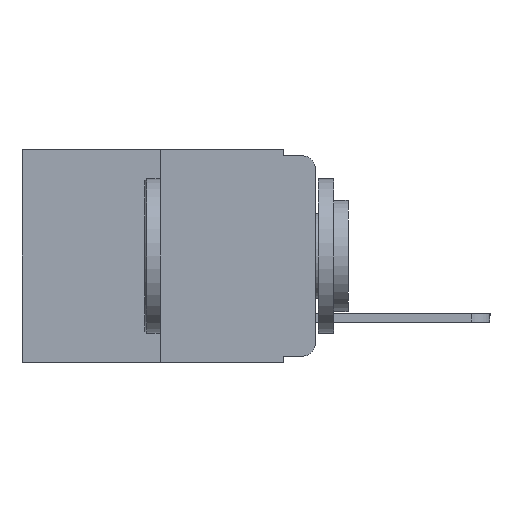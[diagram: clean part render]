
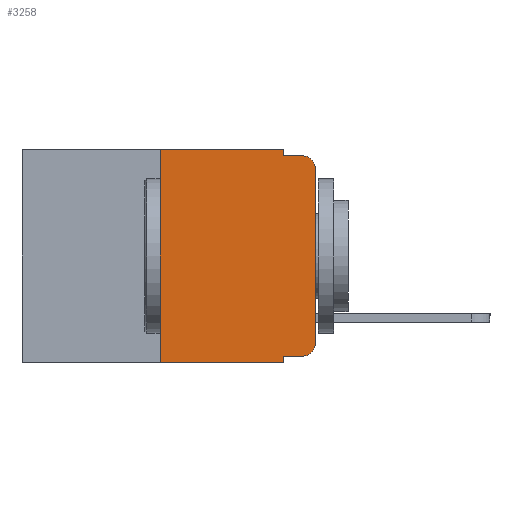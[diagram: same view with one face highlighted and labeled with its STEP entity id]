
A CAD part, left-side view. The second image highlights one B-rep face of the part: STEP entity #3258.
In plain terms, the highlighted planar face has unit normal (-1, 0, 0).
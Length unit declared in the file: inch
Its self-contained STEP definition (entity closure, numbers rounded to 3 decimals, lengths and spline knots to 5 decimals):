
#111 = VECTOR ( 'NONE', #10847, 39.37008 ) ;
#1066 = CARTESIAN_POINT ( 'NONE',  ( 0., 0.051, -0.343 ) ) ;
#1266 = AXIS2_PLACEMENT_3D ( 'NONE', #7223, #21122, #9254 ) ;
#1570 = CARTESIAN_POINT ( 'NONE',  ( 0., 0., -0.03 ) ) ;
#1697 = ORIENTED_EDGE ( 'NONE', *, *, #19129, .T. ) ;
#1716 = DIRECTION ( 'NONE',  ( 0., 0., 1. ) ) ;
#3081 = CARTESIAN_POINT ( 'NONE',  ( 0., 0.051, 0. ) ) ;
#3258 = ADVANCED_FACE ( 'NONE', ( #6547 ), #25032, .F. ) ;
#3435 = LINE ( 'NONE', #7376, #23941 ) ;
#3585 = VECTOR ( 'NONE', #14496, 39.37008 ) ;
#3629 = VECTOR ( 'NONE', #20636, 39.37008 ) ;
#4658 = VERTEX_POINT ( 'NONE', #23649 ) ;
#5950 = VECTOR ( 'NONE', #10369, 39.37008 ) ;
#6118 = ORIENTED_EDGE ( 'NONE', *, *, #22572, .T. ) ;
#6547 = FACE_OUTER_BOUND ( 'NONE', #13446, .T. ) ;
#6591 = CARTESIAN_POINT ( 'NONE',  ( 0., 0.02, -0.01 ) ) ;
#6828 = DIRECTION ( 'NONE',  ( -1., 0., 0. ) ) ;
#6910 = CARTESIAN_POINT ( 'NONE',  ( 0., 0.051, -0.333 ) ) ;
#7209 = AXIS2_PLACEMENT_3D ( 'NONE', #18781, #6828, #20740 ) ;
#7223 = CARTESIAN_POINT ( 'NONE',  ( 0., 0.02, -0.03 ) ) ;
#7250 = EDGE_CURVE ( 'NONE', #8052, #21876, #25751, .T. ) ;
#7376 = CARTESIAN_POINT ( 'NONE',  ( 0., 0.051, -0.333 ) ) ;
#7412 = LINE ( 'NONE', #8847, #111 ) ;
#7690 = ORIENTED_EDGE ( 'NONE', *, *, #24357, .F. ) ;
#7955 = LINE ( 'NONE', #3081, #17935 ) ;
#8052 = VERTEX_POINT ( 'NONE', #14837 ) ;
#8847 = CARTESIAN_POINT ( 'NONE',  ( 0., 0.051, -0.01 ) ) ;
#8939 = LINE ( 'NONE', #10450, #3585 ) ;
#8956 = ORIENTED_EDGE ( 'NONE', *, *, #12789, .F. ) ;
#9242 = DIRECTION ( 'NONE',  ( 0., -1., 0. ) ) ;
#9254 = DIRECTION ( 'NONE',  ( 0., 0., -1. ) ) ;
#9291 = EDGE_CURVE ( 'NONE', #8052, #18500, #14922, .T. ) ;
#9296 = CIRCLE ( 'NONE', #1266, 0.02 ) ;
#10038 = LINE ( 'NONE', #23091, #10674 ) ;
#10175 = ORIENTED_EDGE ( 'NONE', *, *, #10611, .F. ) ;
#10369 = DIRECTION ( 'NONE',  ( 0., -1., 0. ) ) ;
#10387 = VERTEX_POINT ( 'NONE', #17788 ) ;
#10450 = CARTESIAN_POINT ( 'NONE',  ( 0., 0.051, 0. ) ) ;
#10611 = EDGE_CURVE ( 'NONE', #18628, #21876, #8939, .T. ) ;
#10674 = VECTOR ( 'NONE', #9242, 39.37008 ) ;
#10847 = DIRECTION ( 'NONE',  ( 0., -1., 0. ) ) ;
#11144 = LINE ( 'NONE', #13752, #16442 ) ;
#11456 = ORIENTED_EDGE ( 'NONE', *, *, #21250, .T. ) ;
#12789 = EDGE_CURVE ( 'NONE', #18500, #4658, #10038, .T. ) ;
#13200 = CIRCLE ( 'NONE', #7209, 0.02 ) ;
#13446 = EDGE_LOOP ( 'NONE', ( #22276, #1697, #7690, #24114, #8956, #20131, #25324, #10175, #6118, #11456 ) ) ;
#13752 = CARTESIAN_POINT ( 'NONE',  ( 0., 0., 0. ) ) ;
#14496 = DIRECTION ( 'NONE',  ( 0., 0., -1. ) ) ;
#14837 = CARTESIAN_POINT ( 'NONE',  ( 0., 0.25, -0.343 ) ) ;
#14922 = LINE ( 'NONE', #18664, #3629 ) ;
#16130 = VERTEX_POINT ( 'NONE', #6591 ) ;
#16180 = CARTESIAN_POINT ( 'NONE',  ( 0., 0., -0.313 ) ) ;
#16442 = VECTOR ( 'NONE', #1716, 39.37008 ) ;
#16464 = EDGE_CURVE ( 'NONE', #21047, #25197, #11144, .T. ) ;
#16866 = CARTESIAN_POINT ( 'NONE',  ( 0., 0.051, -0.01 ) ) ;
#17788 = CARTESIAN_POINT ( 'NONE',  ( 0., 0.02, -0.333 ) ) ;
#17935 = VECTOR ( 'NONE', #24933, 39.37008 ) ;
#18500 = VERTEX_POINT ( 'NONE', #18513 ) ;
#18513 = CARTESIAN_POINT ( 'NONE',  ( 0., 0.25, 0. ) ) ;
#18628 = VERTEX_POINT ( 'NONE', #6910 ) ;
#18664 = CARTESIAN_POINT ( 'NONE',  ( 0., 0.25, 0. ) ) ;
#18781 = CARTESIAN_POINT ( 'NONE',  ( 0., 0.02, -0.313 ) ) ;
#19129 = EDGE_CURVE ( 'NONE', #25197, #16130, #9296, .T. ) ;
#20131 = ORIENTED_EDGE ( 'NONE', *, *, #9291, .F. ) ;
#20636 = DIRECTION ( 'NONE',  ( 0., 0., 1. ) ) ;
#20740 = DIRECTION ( 'NONE',  ( 0., 0., -1. ) ) ;
#21047 = VERTEX_POINT ( 'NONE', #16180 ) ;
#21122 = DIRECTION ( 'NONE',  ( -1., 0., 0. ) ) ;
#21250 = EDGE_CURVE ( 'NONE', #10387, #21047, #13200, .T. ) ;
#21550 = AXIS2_PLACEMENT_3D ( 'NONE', #23144, #21879, #21911 ) ;
#21876 = VERTEX_POINT ( 'NONE', #1066 ) ;
#21879 = DIRECTION ( 'NONE',  ( 1., 0., 0. ) ) ;
#21911 = DIRECTION ( 'NONE',  ( 0., 0., -1. ) ) ;
#22276 = ORIENTED_EDGE ( 'NONE', *, *, #16464, .T. ) ;
#22572 = EDGE_CURVE ( 'NONE', #18628, #10387, #3435, .T. ) ;
#23091 = CARTESIAN_POINT ( 'NONE',  ( 0., 0.473, 0. ) ) ;
#23144 = CARTESIAN_POINT ( 'NONE',  ( 0., 0.473, 0. ) ) ;
#23249 = DIRECTION ( 'NONE',  ( 0., -1., 0. ) ) ;
#23649 = CARTESIAN_POINT ( 'NONE',  ( 0., 0.051, 0. ) ) ;
#23941 = VECTOR ( 'NONE', #23249, 39.37008 ) ;
#24114 = ORIENTED_EDGE ( 'NONE', *, *, #25647, .F. ) ;
#24202 = CARTESIAN_POINT ( 'NONE',  ( 0., 0.473, -0.343 ) ) ;
#24357 = EDGE_CURVE ( 'NONE', #24376, #16130, #7412, .T. ) ;
#24376 = VERTEX_POINT ( 'NONE', #16866 ) ;
#24933 = DIRECTION ( 'NONE',  ( 0., 0., -1. ) ) ;
#25032 = PLANE ( 'NONE',  #21550 ) ;
#25197 = VERTEX_POINT ( 'NONE', #1570 ) ;
#25324 = ORIENTED_EDGE ( 'NONE', *, *, #7250, .T. ) ;
#25647 = EDGE_CURVE ( 'NONE', #4658, #24376, #7955, .T. ) ;
#25751 = LINE ( 'NONE', #24202, #5950 ) ;
